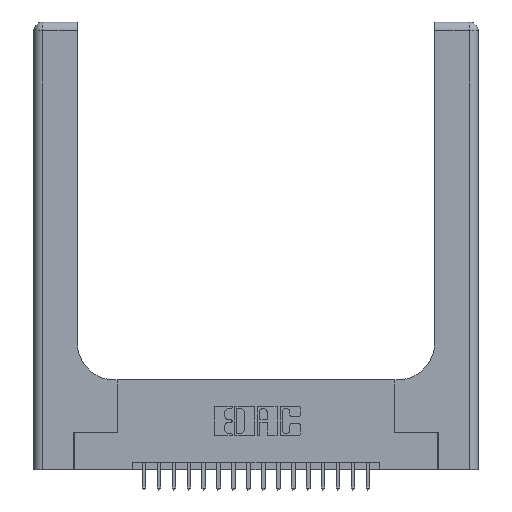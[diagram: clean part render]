
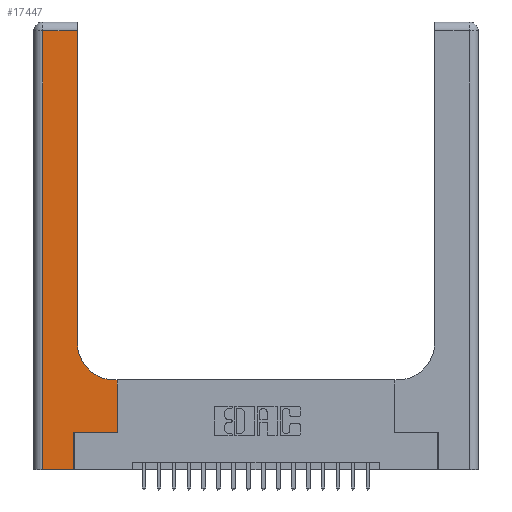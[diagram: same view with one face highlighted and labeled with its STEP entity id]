
A CAD part, top view. The second image highlights one B-rep face of the part: STEP entity #17447.
In plain terms, the highlighted planar face has unit normal (0, 0, 1).
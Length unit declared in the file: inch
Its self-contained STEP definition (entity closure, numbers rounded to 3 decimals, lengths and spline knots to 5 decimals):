
#14 = VECTOR ( 'NONE', #2336, 39.37008 ) ;
#706 = CARTESIAN_POINT ( 'NONE',  ( 0.06, 3., 0.37 ) ) ;
#894 = FACE_OUTER_BOUND ( 'NONE', #11871, .T. ) ;
#966 = DIRECTION ( 'NONE',  ( 1., 0., 0. ) ) ;
#1171 = LINE ( 'NONE', #12898, #3991 ) ;
#1373 = ORIENTED_EDGE ( 'NONE', *, *, #11660, .T. ) ;
#1734 = CARTESIAN_POINT ( 'NONE',  ( 0., 2.94, 0.37 ) ) ;
#2336 = DIRECTION ( 'NONE',  ( 0., 1., 0. ) ) ;
#2822 = DIRECTION ( 'NONE',  ( -1., 0., 0. ) ) ;
#2849 = AXIS2_PLACEMENT_3D ( 'NONE', #13999, #13925, #966 ) ;
#2996 = DIRECTION ( 'NONE',  ( -1., 0., 0. ) ) ;
#3386 = VECTOR ( 'NONE', #2996, 39.37008 ) ;
#3479 = EDGE_CURVE ( 'NONE', #14554, #19609, #14915, .T. ) ;
#3991 = VECTOR ( 'NONE', #9552, 39.37008 ) ;
#4349 = LINE ( 'NONE', #11760, #11518 ) ;
#4429 = LINE ( 'NONE', #19491, #3386 ) ;
#4542 = VERTEX_POINT ( 'NONE', #15898 ) ;
#4910 = EDGE_CURVE ( 'NONE', #5009, #4542, #4349, .T. ) ;
#4928 = DIRECTION ( 'NONE',  ( -1., 0., 0. ) ) ;
#5009 = VERTEX_POINT ( 'NONE', #12184 ) ;
#5125 = CARTESIAN_POINT ( 'NONE',  ( 0.2915, 3., 0.37 ) ) ;
#5774 = EDGE_CURVE ( 'NONE', #19146, #14554, #15254, .T. ) ;
#6314 = ORIENTED_EDGE ( 'NONE', *, *, #12877, .T. ) ;
#6374 = DIRECTION ( 'NONE',  ( 0., 0., -1. ) ) ;
#6720 = LINE ( 'NONE', #1734, #12134 ) ;
#7050 = VECTOR ( 'NONE', #15819, 39.37008 ) ;
#7969 = EDGE_CURVE ( 'NONE', #13980, #16118, #8232, .T. ) ;
#8038 = CARTESIAN_POINT ( 'NONE',  ( 0., 3., 0.37 ) ) ;
#8145 = CARTESIAN_POINT ( 'NONE',  ( 0., 0., 0.37 ) ) ;
#8232 = LINE ( 'NONE', #8145, #16444 ) ;
#8944 = DIRECTION ( 'NONE',  ( 0., -1., 0. ) ) ;
#9348 = LINE ( 'NONE', #12521, #7050 ) ;
#9552 = DIRECTION ( 'NONE',  ( 1., 0., 0. ) ) ;
#9593 = CARTESIAN_POINT ( 'NONE',  ( 0.269, 0.25, 0.37 ) ) ;
#10094 = VERTEX_POINT ( 'NONE', #9593 ) ;
#10963 = CARTESIAN_POINT ( 'NONE',  ( 0.5415, 0.6, 0.37 ) ) ;
#11032 = ORIENTED_EDGE ( 'NONE', *, *, #5774, .T. ) ;
#11518 = VECTOR ( 'NONE', #19878, 39.37008 ) ;
#11660 = EDGE_CURVE ( 'NONE', #10094, #5009, #1171, .T. ) ;
#11760 = CARTESIAN_POINT ( 'NONE',  ( 0.5585, 0.25, 0.37 ) ) ;
#11871 = EDGE_LOOP ( 'NONE', ( #11943, #13180, #6314, #13303, #14741, #1373, #18807, #13040, #11032 ) ) ;
#11943 = ORIENTED_EDGE ( 'NONE', *, *, #3479, .T. ) ;
#12108 = CARTESIAN_POINT ( 'NONE',  ( 0.06, 0., 0.37 ) ) ;
#12134 = VECTOR ( 'NONE', #4928, 39.37008 ) ;
#12184 = CARTESIAN_POINT ( 'NONE',  ( 0.5585, 0.25, 0.37 ) ) ;
#12521 = CARTESIAN_POINT ( 'NONE',  ( 0.269, 0., 0.37 ) ) ;
#12877 = EDGE_CURVE ( 'NONE', #20813, #13980, #20299, .T. ) ;
#12898 = CARTESIAN_POINT ( 'NONE',  ( 0.269, 0.25, 0.37 ) ) ;
#13040 = ORIENTED_EDGE ( 'NONE', *, *, #18729, .T. ) ;
#13180 = ORIENTED_EDGE ( 'NONE', *, *, #18172, .T. ) ;
#13303 = ORIENTED_EDGE ( 'NONE', *, *, #7969, .T. ) ;
#13636 = CARTESIAN_POINT ( 'NONE',  ( 0.2915, 2.94, 0.37 ) ) ;
#13925 = DIRECTION ( 'NONE',  ( 0., 0., -1. ) ) ;
#13980 = VERTEX_POINT ( 'NONE', #12108 ) ;
#13999 = CARTESIAN_POINT ( 'NONE',  ( 0.5415, 0.85, 0.37 ) ) ;
#14554 = VERTEX_POINT ( 'NONE', #18443 ) ;
#14741 = ORIENTED_EDGE ( 'NONE', *, *, #19235, .T. ) ;
#14915 = LINE ( 'NONE', #5125, #14 ) ;
#15254 = CIRCLE ( 'NONE', #2849, 0.25 ) ;
#15819 = DIRECTION ( 'NONE',  ( 0., 1., 0. ) ) ;
#15856 = CARTESIAN_POINT ( 'NONE',  ( 0.06, 2.94, 0.37 ) ) ;
#15898 = CARTESIAN_POINT ( 'NONE',  ( 0.5585, 0.6, 0.37 ) ) ;
#16004 = PLANE ( 'NONE',  #18663 ) ;
#16118 = VERTEX_POINT ( 'NONE', #17267 ) ;
#16404 = DIRECTION ( 'NONE',  ( 1., 0., 0. ) ) ;
#16444 = VECTOR ( 'NONE', #16404, 39.37008 ) ;
#16948 = VECTOR ( 'NONE', #8944, 39.37008 ) ;
#17267 = CARTESIAN_POINT ( 'NONE',  ( 0.269, 0., 0.37 ) ) ;
#17447 = ADVANCED_FACE ( 'NONE', ( #894 ), #16004, .F. ) ;
#18172 = EDGE_CURVE ( 'NONE', #19609, #20813, #6720, .T. ) ;
#18443 = CARTESIAN_POINT ( 'NONE',  ( 0.2915, 0.85, 0.37 ) ) ;
#18663 = AXIS2_PLACEMENT_3D ( 'NONE', #8038, #6374, #2822 ) ;
#18729 = EDGE_CURVE ( 'NONE', #4542, #19146, #4429, .T. ) ;
#18807 = ORIENTED_EDGE ( 'NONE', *, *, #4910, .T. ) ;
#19146 = VERTEX_POINT ( 'NONE', #10963 ) ;
#19235 = EDGE_CURVE ( 'NONE', #16118, #10094, #9348, .T. ) ;
#19491 = CARTESIAN_POINT ( 'NONE',  ( 0.2915, 0.6, 0.37 ) ) ;
#19609 = VERTEX_POINT ( 'NONE', #13636 ) ;
#19878 = DIRECTION ( 'NONE',  ( 0., 1., 0. ) ) ;
#20299 = LINE ( 'NONE', #706, #16948 ) ;
#20813 = VERTEX_POINT ( 'NONE', #15856 ) ;
